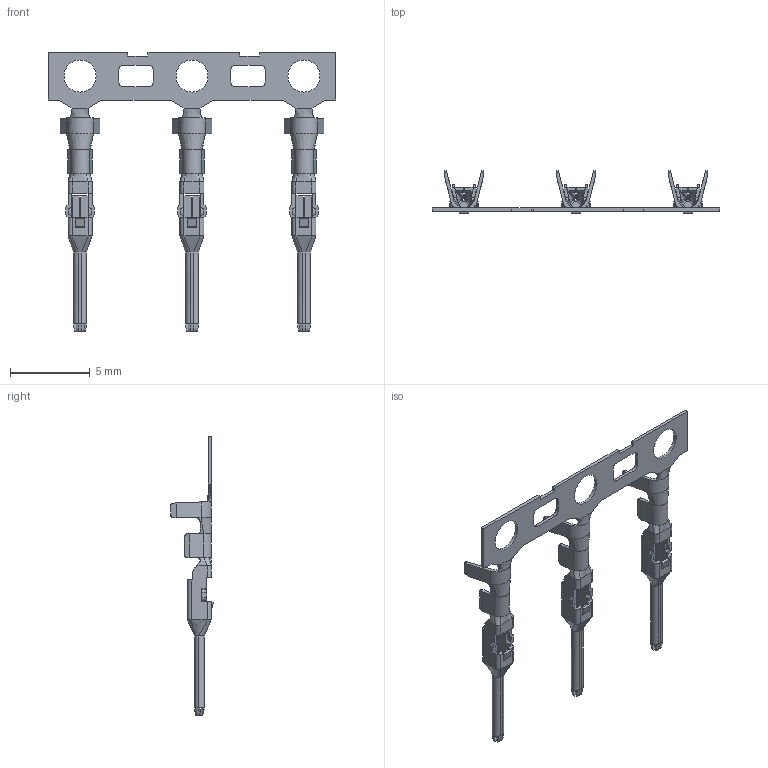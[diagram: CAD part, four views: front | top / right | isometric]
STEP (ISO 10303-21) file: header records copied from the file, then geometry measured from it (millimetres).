
FILE_DESCRIPTION (( 'STEP AP214' ), '1' );
FILE_NAME ('565-290-711 STRIP.STEP', '2020-09-17T17:26:19', ( '' ), ( '' ), 'SwSTEP 2.0', 'SolidWorks 2020', '' );
FILE_SCHEMA (( 'AUTOMOTIVE_DESIGN' ));
Length unit declared in the file: millimetre
Products named in the file (3): 565-290-711 STRIP; 565-290-711; 565-290-711_CARRIER-STRIP
Assembly tree (4 placements, depth 2):
  565-290-711 STRIP
    565-290-711_CARRIER-STRIP
    565-290-711  x3
Bounding box: 18 x 2.68 x 17.5 mm (x, y, z)
Volume: 30.4 mm3; surface area: 362.5 mm2
Topology: 7 solids, 7 shells, 778 faces, 2100 edges, 1330 vertices
Faces by surface type: plane 374, cylinder 257, bspline 108, torus 21, cone 18
Entity records: 11158 total; most frequent: CARTESIAN_POINT 3843, ORIENTED_EDGE 1620, DIRECTION 1315, EDGE_CURVE 810, VERTEX_POINT 514, LINE 499, VECTOR 499, AXIS2_PLACEMENT_3D 408
